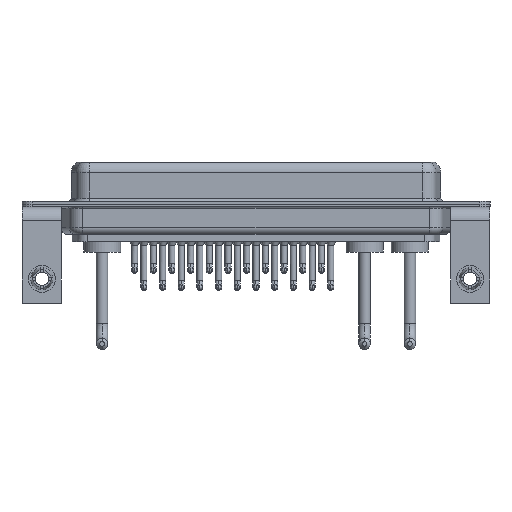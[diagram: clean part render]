
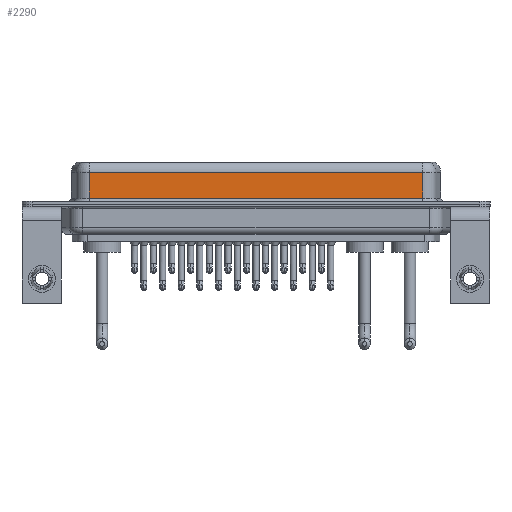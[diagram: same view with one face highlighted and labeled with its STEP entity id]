
A CAD part, front view. The second image highlights one B-rep face of the part: STEP entity #2290.
In plain terms, the highlighted planar face has unit normal (0, -1, 0).
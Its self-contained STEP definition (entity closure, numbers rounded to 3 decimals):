
#325 = LINE ( 'NONE', #7672, #3058 ) ;
#1479 = ORIENTED_EDGE ( 'NONE', *, *, #15527, .T. ) ;
#2290 = ADVANCED_FACE ( 'NONE', ( #6890 ), #21089, .F. ) ;
#2415 = VECTOR ( 'NONE', #18819, 1000. ) ;
#3058 = VECTOR ( 'NONE', #13903, 1000. ) ;
#3589 = VECTOR ( 'NONE', #24211, 1000. ) ;
#6890 = FACE_OUTER_BOUND ( 'NONE', #9152, .T. ) ;
#7158 = CARTESIAN_POINT ( 'NONE',  ( 56.462, -3.95, 6.4 ) ) ;
#7164 = ORIENTED_EDGE ( 'NONE', *, *, #19331, .T. ) ;
#7486 = AXIS2_PLACEMENT_3D ( 'NONE', #7158, #15276, #15788 ) ;
#7672 = CARTESIAN_POINT ( 'NONE',  ( 56.462, -3.95, 0.9 ) ) ;
#8903 = VERTEX_POINT ( 'NONE', #24679 ) ;
#8985 = VERTEX_POINT ( 'NONE', #10251 ) ;
#9152 = EDGE_LOOP ( 'NONE', ( #19627, #1479, #18165, #7164 ) ) ;
#9180 = LINE ( 'NONE', #25204, #22285 ) ;
#9661 = LINE ( 'NONE', #22254, #3589 ) ;
#10251 = CARTESIAN_POINT ( 'NONE',  ( 7.038, -3.95, 4.65 ) ) ;
#11185 = DIRECTION ( 'NONE',  ( -1., 0., 0. ) ) ;
#12457 = VERTEX_POINT ( 'NONE', #23984 ) ;
#12967 = EDGE_CURVE ( 'NONE', #24243, #8903, #9661, .T. ) ;
#13903 = DIRECTION ( 'NONE',  ( 1., 0., 0. ) ) ;
#15276 = DIRECTION ( 'NONE',  ( 0., 1., 0. ) ) ;
#15527 = EDGE_CURVE ( 'NONE', #24243, #8985, #9180, .T. ) ;
#15726 = CARTESIAN_POINT ( 'NONE',  ( 56.462, -3.95, 4.65 ) ) ;
#15788 = DIRECTION ( 'NONE',  ( 0., 0., 1. ) ) ;
#18165 = ORIENTED_EDGE ( 'NONE', *, *, #24839, .T. ) ;
#18819 = DIRECTION ( 'NONE',  ( 0., 0., -1. ) ) ;
#19331 = EDGE_CURVE ( 'NONE', #12457, #8903, #325, .T. ) ;
#19627 = ORIENTED_EDGE ( 'NONE', *, *, #12967, .F. ) ;
#20785 = CARTESIAN_POINT ( 'NONE',  ( 7.038, -3.95, 6.4 ) ) ;
#21089 = PLANE ( 'NONE',  #7486 ) ;
#22254 = CARTESIAN_POINT ( 'NONE',  ( 56.462, -3.95, 6.4 ) ) ;
#22285 = VECTOR ( 'NONE', #11185, 1000. ) ;
#22906 = LINE ( 'NONE', #20785, #2415 ) ;
#23984 = CARTESIAN_POINT ( 'NONE',  ( 7.038, -3.95, 0.9 ) ) ;
#24211 = DIRECTION ( 'NONE',  ( 0., 0., -1. ) ) ;
#24243 = VERTEX_POINT ( 'NONE', #15726 ) ;
#24679 = CARTESIAN_POINT ( 'NONE',  ( 56.462, -3.95, 0.9 ) ) ;
#24839 = EDGE_CURVE ( 'NONE', #8985, #12457, #22906, .T. ) ;
#25204 = CARTESIAN_POINT ( 'NONE',  ( 56.462, -3.95, 4.65 ) ) ;
